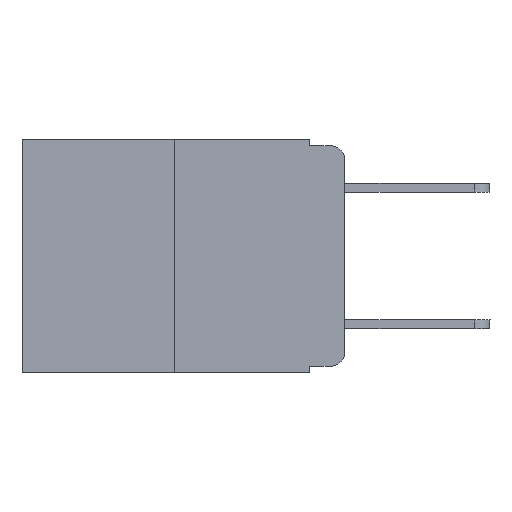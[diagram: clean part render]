
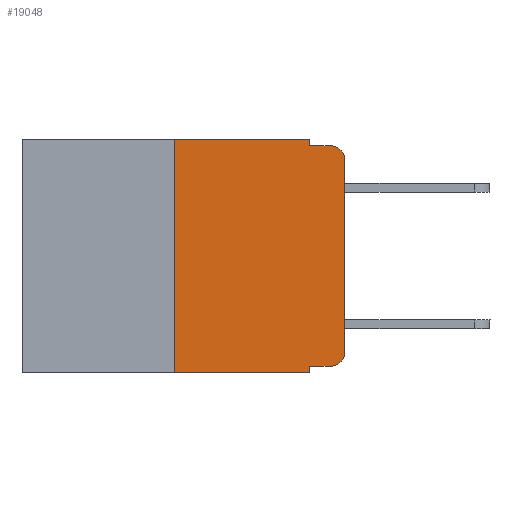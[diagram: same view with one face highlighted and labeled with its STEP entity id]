
A CAD part, left-side view. The second image highlights one B-rep face of the part: STEP entity #19048.
In plain terms, the highlighted planar face has unit normal (-1, 0, 0).
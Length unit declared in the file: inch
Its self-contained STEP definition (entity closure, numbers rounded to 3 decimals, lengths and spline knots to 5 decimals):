
#44 = VECTOR ( 'NONE', #22567, 39.37008 ) ;
#58 = LINE ( 'NONE', #13412, #20400 ) ;
#1665 = CARTESIAN_POINT ( 'NONE',  ( 0., 0.051, -0.333 ) ) ;
#1732 = VERTEX_POINT ( 'NONE', #14424 ) ;
#1790 = EDGE_CURVE ( 'NONE', #23813, #11533, #20059, .T. ) ;
#2030 = CARTESIAN_POINT ( 'NONE',  ( 0., 0., -0.313 ) ) ;
#2091 = DIRECTION ( 'NONE',  ( -1., 0., 0. ) ) ;
#2214 = EDGE_CURVE ( 'NONE', #10120, #23813, #15130, .T. ) ;
#2216 = ORIENTED_EDGE ( 'NONE', *, *, #19096, .T. ) ;
#2471 = VERTEX_POINT ( 'NONE', #19379 ) ;
#2888 = VECTOR ( 'NONE', #12551, 39.37008 ) ;
#2977 = CARTESIAN_POINT ( 'NONE',  ( 0., 0.473, -0.343 ) ) ;
#3569 = VECTOR ( 'NONE', #14919, 39.37008 ) ;
#3686 = AXIS2_PLACEMENT_3D ( 'NONE', #9988, #17626, #15742 ) ;
#4971 = EDGE_CURVE ( 'NONE', #23735, #18525, #20109, .T. ) ;
#5417 = DIRECTION ( 'NONE',  ( 0., 0., 1. ) ) ;
#6354 = DIRECTION ( 'NONE',  ( 0., 0., -1. ) ) ;
#6889 = CIRCLE ( 'NONE', #3686, 0.02 ) ;
#6979 = EDGE_CURVE ( 'NONE', #15793, #23735, #16928, .T. ) ;
#7114 = CARTESIAN_POINT ( 'NONE',  ( 0., 0.051, -0.333 ) ) ;
#7371 = EDGE_LOOP ( 'NONE', ( #24475, #2216, #20413, #21852, #16996, #13626, #19826, #11388, #12510, #20531 ) ) ;
#7404 = CARTESIAN_POINT ( 'NONE',  ( 0., 0.473, 0. ) ) ;
#8122 = DIRECTION ( 'NONE',  ( 1., 0., 0. ) ) ;
#9797 = CARTESIAN_POINT ( 'NONE',  ( 0., 0., 0. ) ) ;
#9988 = CARTESIAN_POINT ( 'NONE',  ( 0., 0.02, -0.03 ) ) ;
#10120 = VERTEX_POINT ( 'NONE', #16814 ) ;
#10289 = VECTOR ( 'NONE', #22902, 39.37008 ) ;
#10968 = LINE ( 'NONE', #2977, #22386 ) ;
#11388 = ORIENTED_EDGE ( 'NONE', *, *, #11481, .F. ) ;
#11449 = EDGE_CURVE ( 'NONE', #1732, #10120, #18811, .T. ) ;
#11481 = EDGE_CURVE ( 'NONE', #15793, #2471, #13029, .T. ) ;
#11533 = VERTEX_POINT ( 'NONE', #24313 ) ;
#11564 = LINE ( 'NONE', #9797, #44 ) ;
#11619 = CARTESIAN_POINT ( 'NONE',  ( 0., 0.02, -0.333 ) ) ;
#11636 = FACE_OUTER_BOUND ( 'NONE', #7371, .T. ) ;
#11696 = DIRECTION ( 'NONE',  ( 0., -1., 0. ) ) ;
#12510 = ORIENTED_EDGE ( 'NONE', *, *, #6979, .T. ) ;
#12551 = DIRECTION ( 'NONE',  ( 0., 0., -1. ) ) ;
#12789 = CARTESIAN_POINT ( 'NONE',  ( 0., 0.25, 0. ) ) ;
#12847 = VERTEX_POINT ( 'NONE', #23608 ) ;
#13029 = LINE ( 'NONE', #22172, #3569 ) ;
#13412 = CARTESIAN_POINT ( 'NONE',  ( 0., 0.051, -0.01 ) ) ;
#13626 = ORIENTED_EDGE ( 'NONE', *, *, #11449, .F. ) ;
#13942 = VECTOR ( 'NONE', #5417, 39.37008 ) ;
#14202 = CARTESIAN_POINT ( 'NONE',  ( 0., 0., -0.03 ) ) ;
#14318 = EDGE_CURVE ( 'NONE', #1732, #2471, #10968, .T. ) ;
#14424 = CARTESIAN_POINT ( 'NONE',  ( 0., 0.25, -0.343 ) ) ;
#14579 = DIRECTION ( 'NONE',  ( 0., -1., 0. ) ) ;
#14919 = DIRECTION ( 'NONE',  ( 0., 0., -1. ) ) ;
#15130 = LINE ( 'NONE', #7404, #10289 ) ;
#15560 = VECTOR ( 'NONE', #20782, 39.37008 ) ;
#15742 = DIRECTION ( 'NONE',  ( 0., 0., -1. ) ) ;
#15793 = VERTEX_POINT ( 'NONE', #7114 ) ;
#16074 = AXIS2_PLACEMENT_3D ( 'NONE', #21255, #8122, #6354 ) ;
#16814 = CARTESIAN_POINT ( 'NONE',  ( 0., 0.25, 0. ) ) ;
#16928 = LINE ( 'NONE', #1665, #15560 ) ;
#16996 = ORIENTED_EDGE ( 'NONE', *, *, #2214, .F. ) ;
#17626 = DIRECTION ( 'NONE',  ( -1., 0., 0. ) ) ;
#18041 = EDGE_CURVE ( 'NONE', #18525, #19747, #11564, .T. ) ;
#18056 = EDGE_CURVE ( 'NONE', #11533, #12847, #58, .T. ) ;
#18525 = VERTEX_POINT ( 'NONE', #2030 ) ;
#18811 = LINE ( 'NONE', #12789, #13942 ) ;
#19048 = ADVANCED_FACE ( 'NONE', ( #11636 ), #19366, .F. ) ;
#19096 = EDGE_CURVE ( 'NONE', #19747, #12847, #6889, .T. ) ;
#19215 = DIRECTION ( 'NONE',  ( 0., 0., -1. ) ) ;
#19366 = PLANE ( 'NONE',  #16074 ) ;
#19379 = CARTESIAN_POINT ( 'NONE',  ( 0., 0.051, -0.343 ) ) ;
#19747 = VERTEX_POINT ( 'NONE', #14202 ) ;
#19826 = ORIENTED_EDGE ( 'NONE', *, *, #14318, .T. ) ;
#20059 = LINE ( 'NONE', #22060, #2888 ) ;
#20109 = CIRCLE ( 'NONE', #23321, 0.02 ) ;
#20400 = VECTOR ( 'NONE', #11696, 39.37008 ) ;
#20413 = ORIENTED_EDGE ( 'NONE', *, *, #18056, .F. ) ;
#20531 = ORIENTED_EDGE ( 'NONE', *, *, #4971, .T. ) ;
#20782 = DIRECTION ( 'NONE',  ( 0., -1., 0. ) ) ;
#21255 = CARTESIAN_POINT ( 'NONE',  ( 0., 0.473, 0. ) ) ;
#21852 = ORIENTED_EDGE ( 'NONE', *, *, #1790, .F. ) ;
#22060 = CARTESIAN_POINT ( 'NONE',  ( 0., 0.051, 0. ) ) ;
#22172 = CARTESIAN_POINT ( 'NONE',  ( 0., 0.051, 0. ) ) ;
#22386 = VECTOR ( 'NONE', #14579, 39.37008 ) ;
#22567 = DIRECTION ( 'NONE',  ( 0., 0., 1. ) ) ;
#22902 = DIRECTION ( 'NONE',  ( 0., -1., 0. ) ) ;
#22977 = CARTESIAN_POINT ( 'NONE',  ( 0., 0.02, -0.313 ) ) ;
#23321 = AXIS2_PLACEMENT_3D ( 'NONE', #22977, #2091, #19215 ) ;
#23608 = CARTESIAN_POINT ( 'NONE',  ( 0., 0.02, -0.01 ) ) ;
#23735 = VERTEX_POINT ( 'NONE', #11619 ) ;
#23813 = VERTEX_POINT ( 'NONE', #23853 ) ;
#23853 = CARTESIAN_POINT ( 'NONE',  ( 0., 0.051, 0. ) ) ;
#24313 = CARTESIAN_POINT ( 'NONE',  ( 0., 0.051, -0.01 ) ) ;
#24475 = ORIENTED_EDGE ( 'NONE', *, *, #18041, .T. ) ;
